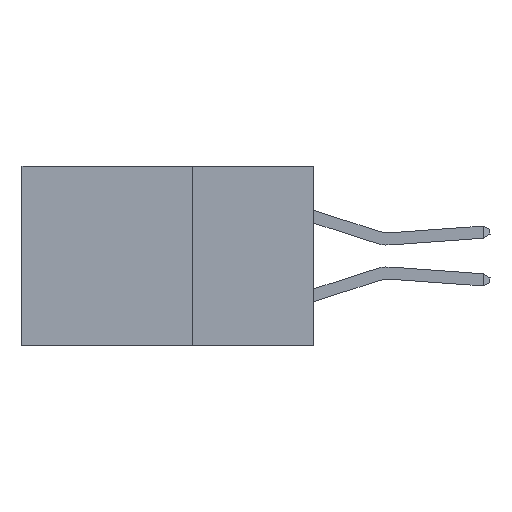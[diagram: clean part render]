
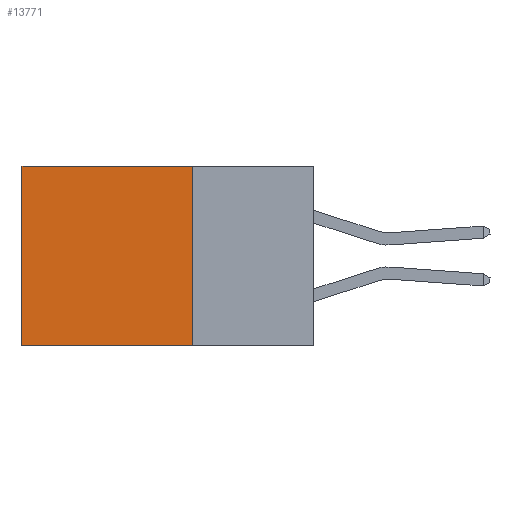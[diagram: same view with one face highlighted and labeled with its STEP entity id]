
A CAD part, left-side view. The second image highlights one B-rep face of the part: STEP entity #13771.
In plain terms, the highlighted planar face has unit normal (-1, 0, 0).
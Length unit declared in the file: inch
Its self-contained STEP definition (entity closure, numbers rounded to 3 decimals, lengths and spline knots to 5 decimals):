
#190 = CARTESIAN_POINT ( 'NONE',  ( 0.2875, 0.25, 0. ) ) ;
#418 = LINE ( 'NONE', #14120, #8497 ) ;
#473 = ORIENTED_EDGE ( 'NONE', *, *, #8777, .F. ) ;
#844 = CARTESIAN_POINT ( 'NONE',  ( 0.2875, 0.6, -0.37 ) ) ;
#1104 = AXIS2_PLACEMENT_3D ( 'NONE', #190, #1262, #12095 ) ;
#1249 = DIRECTION ( 'NONE',  ( 0., 1., 0. ) ) ;
#1262 = DIRECTION ( 'NONE',  ( 1., 0., 0. ) ) ;
#1632 = VECTOR ( 'NONE', #14239, 39.37008 ) ;
#1964 = LINE ( 'NONE', #13209, #5399 ) ;
#2386 = VERTEX_POINT ( 'NONE', #11042 ) ;
#4771 = CARTESIAN_POINT ( 'NONE',  ( 0.2875, 0.25, 0. ) ) ;
#4784 = EDGE_CURVE ( 'NONE', #13036, #2386, #1964, .T. ) ;
#5399 = VECTOR ( 'NONE', #1249, 39.37008 ) ;
#5430 = CARTESIAN_POINT ( 'NONE',  ( 0.2875, 0.25, -0.37 ) ) ;
#5807 = ORIENTED_EDGE ( 'NONE', *, *, #5814, .F. ) ;
#5814 = EDGE_CURVE ( 'NONE', #13036, #9721, #13877, .T. ) ;
#5985 = CARTESIAN_POINT ( 'NONE',  ( 0.2875, 0.25, -0.37 ) ) ;
#7137 = CARTESIAN_POINT ( 'NONE',  ( 0.2875, 0.25, 0. ) ) ;
#8229 = VERTEX_POINT ( 'NONE', #844 ) ;
#8354 = EDGE_LOOP ( 'NONE', ( #13295, #473, #5807, #10511 ) ) ;
#8497 = VECTOR ( 'NONE', #15210, 39.37008 ) ;
#8777 = EDGE_CURVE ( 'NONE', #9721, #8229, #15494, .T. ) ;
#9721 = VERTEX_POINT ( 'NONE', #5430 ) ;
#10511 = ORIENTED_EDGE ( 'NONE', *, *, #4784, .T. ) ;
#11042 = CARTESIAN_POINT ( 'NONE',  ( 0.2875, 0.6, 0. ) ) ;
#12052 = PLANE ( 'NONE',  #1104 ) ;
#12095 = DIRECTION ( 'NONE',  ( 0., 0., -1. ) ) ;
#12239 = EDGE_CURVE ( 'NONE', #2386, #8229, #418, .T. ) ;
#13036 = VERTEX_POINT ( 'NONE', #7137 ) ;
#13209 = CARTESIAN_POINT ( 'NONE',  ( 0.2875, 0.25, 0. ) ) ;
#13295 = ORIENTED_EDGE ( 'NONE', *, *, #12239, .T. ) ;
#13771 = ADVANCED_FACE ( 'NONE', ( #13804 ), #12052, .F. ) ;
#13804 = FACE_OUTER_BOUND ( 'NONE', #8354, .T. ) ;
#13877 = LINE ( 'NONE', #4771, #14635 ) ;
#14120 = CARTESIAN_POINT ( 'NONE',  ( 0.2875, 0.6, 0. ) ) ;
#14239 = DIRECTION ( 'NONE',  ( 0., 1., 0. ) ) ;
#14635 = VECTOR ( 'NONE', #15484, 39.37008 ) ;
#15210 = DIRECTION ( 'NONE',  ( 0., 0., -1. ) ) ;
#15484 = DIRECTION ( 'NONE',  ( 0., 0., -1. ) ) ;
#15494 = LINE ( 'NONE', #5985, #1632 ) ;
